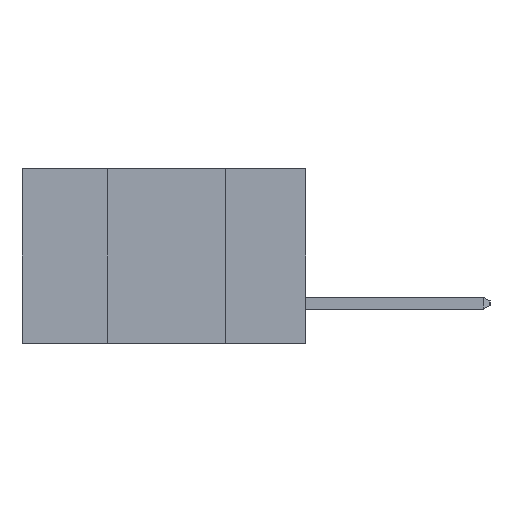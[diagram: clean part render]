
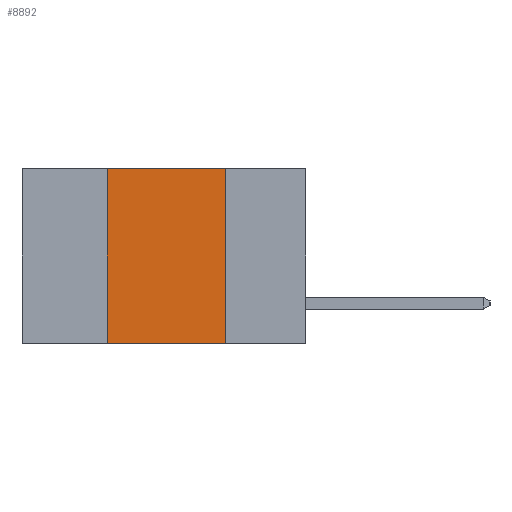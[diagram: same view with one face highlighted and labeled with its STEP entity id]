
A CAD part, left-side view. The second image highlights one B-rep face of the part: STEP entity #8892.
In plain terms, the highlighted planar face has unit normal (-1, 0, 0).
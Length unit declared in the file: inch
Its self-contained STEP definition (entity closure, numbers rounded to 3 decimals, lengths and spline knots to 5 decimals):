
#489 = LINE ( 'NONE', #2144, #6639 ) ;
#498 = PLANE ( 'NONE',  #2056 ) ;
#691 = CARTESIAN_POINT ( 'NONE',  ( 0., 0.6, 0. ) ) ;
#1016 = EDGE_CURVE ( 'NONE', #6685, #3522, #7813, .T. ) ;
#1166 = VECTOR ( 'NONE', #5893, 39.37008 ) ;
#2056 = AXIS2_PLACEMENT_3D ( 'NONE', #6494, #7284, #2364 ) ;
#2144 = CARTESIAN_POINT ( 'NONE',  ( 0., 0.42, -0.37 ) ) ;
#2364 = DIRECTION ( 'NONE',  ( 0., 0., -1. ) ) ;
#2554 = CARTESIAN_POINT ( 'NONE',  ( 0., 0.42, 0. ) ) ;
#2633 = VECTOR ( 'NONE', #8367, 39.37008 ) ;
#3264 = EDGE_CURVE ( 'NONE', #6435, #9776, #489, .T. ) ;
#3472 = ORIENTED_EDGE ( 'NONE', *, *, #8333, .F. ) ;
#3522 = VERTEX_POINT ( 'NONE', #8977 ) ;
#3588 = LINE ( 'NONE', #691, #7614 ) ;
#3852 = EDGE_CURVE ( 'NONE', #6435, #3522, #8889, .T. ) ;
#4008 = CARTESIAN_POINT ( 'NONE',  ( 0., 0.42, -0.37 ) ) ;
#4244 = CARTESIAN_POINT ( 'NONE',  ( 0., 0.17, -0.37 ) ) ;
#5019 = ORIENTED_EDGE ( 'NONE', *, *, #3852, .T. ) ;
#5481 = FACE_OUTER_BOUND ( 'NONE', #8758, .T. ) ;
#5893 = DIRECTION ( 'NONE',  ( 0., 0., -1. ) ) ;
#6012 = ORIENTED_EDGE ( 'NONE', *, *, #3264, .F. ) ;
#6435 = VERTEX_POINT ( 'NONE', #4008 ) ;
#6494 = CARTESIAN_POINT ( 'NONE',  ( 0., 0.6, 0. ) ) ;
#6616 = CARTESIAN_POINT ( 'NONE',  ( 0., 0.17, 0. ) ) ;
#6639 = VECTOR ( 'NONE', #7120, 39.37008 ) ;
#6685 = VERTEX_POINT ( 'NONE', #6616 ) ;
#7120 = DIRECTION ( 'NONE',  ( 0., 0., 1. ) ) ;
#7284 = DIRECTION ( 'NONE',  ( 1., 0., 0. ) ) ;
#7614 = VECTOR ( 'NONE', #8199, 39.37008 ) ;
#7734 = ORIENTED_EDGE ( 'NONE', *, *, #1016, .F. ) ;
#7813 = LINE ( 'NONE', #4244, #1166 ) ;
#8199 = DIRECTION ( 'NONE',  ( 0., -1., 0. ) ) ;
#8333 = EDGE_CURVE ( 'NONE', #9776, #6685, #3588, .T. ) ;
#8367 = DIRECTION ( 'NONE',  ( 0., -1., 0. ) ) ;
#8390 = CARTESIAN_POINT ( 'NONE',  ( 0., 0.6, -0.37 ) ) ;
#8758 = EDGE_LOOP ( 'NONE', ( #7734, #3472, #6012, #5019 ) ) ;
#8889 = LINE ( 'NONE', #8390, #2633 ) ;
#8892 = ADVANCED_FACE ( 'NONE', ( #5481 ), #498, .F. ) ;
#8977 = CARTESIAN_POINT ( 'NONE',  ( 0., 0.17, -0.37 ) ) ;
#9776 = VERTEX_POINT ( 'NONE', #2554 ) ;
